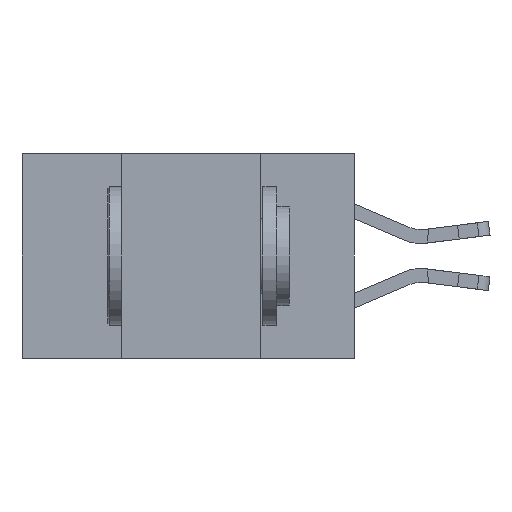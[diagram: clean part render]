
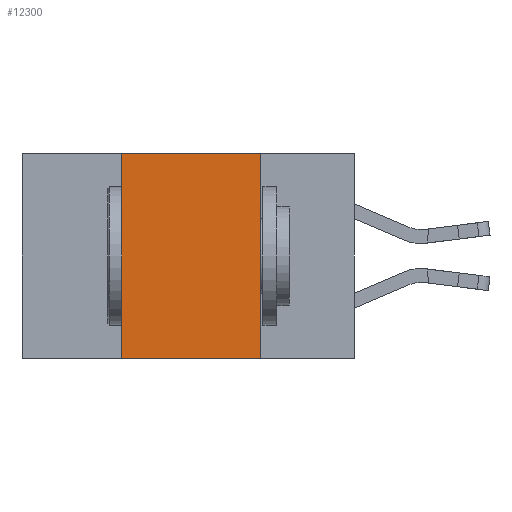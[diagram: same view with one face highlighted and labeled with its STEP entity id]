
A CAD part, left-side view. The second image highlights one B-rep face of the part: STEP entity #12300.
In plain terms, the highlighted planar face has unit normal (-1, 0, 0).
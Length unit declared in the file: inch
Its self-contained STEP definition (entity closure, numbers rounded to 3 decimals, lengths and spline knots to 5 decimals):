
#1156 = CARTESIAN_POINT ( 'NONE',  ( 0., 0.17, 0. ) ) ;
#1400 = EDGE_CURVE ( 'NONE', #8507, #3274, #7834, .T. ) ;
#1542 = PLANE ( 'NONE',  #8083 ) ;
#1669 = DIRECTION ( 'NONE',  ( 0., 0., 1. ) ) ;
#2366 = VECTOR ( 'NONE', #14942, 39.37008 ) ;
#2531 = LINE ( 'NONE', #11010, #10648 ) ;
#3217 = VERTEX_POINT ( 'NONE', #11290 ) ;
#3274 = VERTEX_POINT ( 'NONE', #11426 ) ;
#4253 = ORIENTED_EDGE ( 'NONE', *, *, #1400, .T. ) ;
#4741 = VECTOR ( 'NONE', #7900, 39.37008 ) ;
#6196 = EDGE_CURVE ( 'NONE', #3217, #14570, #14122, .T. ) ;
#6586 = EDGE_CURVE ( 'NONE', #8507, #3217, #2531, .T. ) ;
#7324 = CARTESIAN_POINT ( 'NONE',  ( 0., 0.6, 0. ) ) ;
#7834 = LINE ( 'NONE', #14377, #4741 ) ;
#7900 = DIRECTION ( 'NONE',  ( 0., -1., 0. ) ) ;
#8083 = AXIS2_PLACEMENT_3D ( 'NONE', #7324, #8792, #8745 ) ;
#8346 = ORIENTED_EDGE ( 'NONE', *, *, #6196, .F. ) ;
#8465 = CARTESIAN_POINT ( 'NONE',  ( 0., 0.17, 0. ) ) ;
#8507 = VERTEX_POINT ( 'NONE', #13710 ) ;
#8745 = DIRECTION ( 'NONE',  ( 0., 0., -1. ) ) ;
#8792 = DIRECTION ( 'NONE',  ( 1., 0., 0. ) ) ;
#9025 = FACE_OUTER_BOUND ( 'NONE', #10472, .T. ) ;
#9234 = LINE ( 'NONE', #1156, #2366 ) ;
#10472 = EDGE_LOOP ( 'NONE', ( #11879, #8346, #12252, #4253 ) ) ;
#10648 = VECTOR ( 'NONE', #1669, 39.37008 ) ;
#11010 = CARTESIAN_POINT ( 'NONE',  ( 0., 0.42, 0. ) ) ;
#11182 = CARTESIAN_POINT ( 'NONE',  ( 0., 0.6, 0. ) ) ;
#11290 = CARTESIAN_POINT ( 'NONE',  ( 0., 0.42, 0. ) ) ;
#11426 = CARTESIAN_POINT ( 'NONE',  ( 0., 0.17, -0.37 ) ) ;
#11591 = EDGE_CURVE ( 'NONE', #14570, #3274, #9234, .T. ) ;
#11879 = ORIENTED_EDGE ( 'NONE', *, *, #11591, .F. ) ;
#11940 = VECTOR ( 'NONE', #14566, 39.37008 ) ;
#12252 = ORIENTED_EDGE ( 'NONE', *, *, #6586, .F. ) ;
#12300 = ADVANCED_FACE ( 'NONE', ( #9025 ), #1542, .F. ) ;
#13710 = CARTESIAN_POINT ( 'NONE',  ( 0., 0.42, -0.37 ) ) ;
#14122 = LINE ( 'NONE', #11182, #11940 ) ;
#14377 = CARTESIAN_POINT ( 'NONE',  ( 0., 0.6, -0.37 ) ) ;
#14566 = DIRECTION ( 'NONE',  ( 0., -1., 0. ) ) ;
#14570 = VERTEX_POINT ( 'NONE', #8465 ) ;
#14942 = DIRECTION ( 'NONE',  ( 0., 0., -1. ) ) ;
